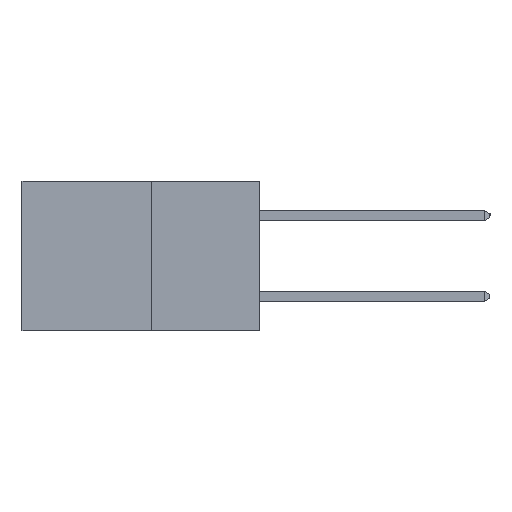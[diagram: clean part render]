
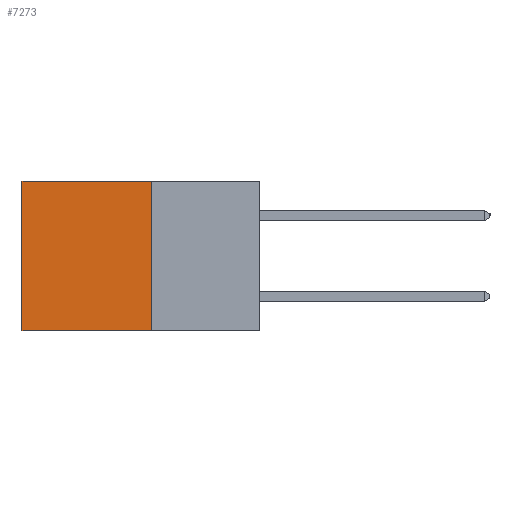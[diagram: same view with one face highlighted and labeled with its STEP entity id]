
A CAD part, left-side view. The second image highlights one B-rep face of the part: STEP entity #7273.
In plain terms, the highlighted planar face has unit normal (-1, 0, 0).
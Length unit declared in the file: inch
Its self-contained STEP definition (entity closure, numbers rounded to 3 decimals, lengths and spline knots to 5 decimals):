
#501 = LINE ( 'NONE', #6495, #8125 ) ;
#577 = VERTEX_POINT ( 'NONE', #7725 ) ;
#674 = ORIENTED_EDGE ( 'NONE', *, *, #4969, .F. ) ;
#1508 = LINE ( 'NONE', #6036, #3295 ) ;
#1708 = FACE_OUTER_BOUND ( 'NONE', #6124, .T. ) ;
#1887 = CARTESIAN_POINT ( 'NONE',  ( 0.277, 0.27, -0.37 ) ) ;
#2261 = CARTESIAN_POINT ( 'NONE',  ( 0.277, 0.27, 0. ) ) ;
#2389 = ORIENTED_EDGE ( 'NONE', *, *, #8912, .T. ) ;
#2545 = VERTEX_POINT ( 'NONE', #6766 ) ;
#2598 = DIRECTION ( 'NONE',  ( 1., 0., 0. ) ) ;
#2886 = PLANE ( 'NONE',  #6921 ) ;
#3295 = VECTOR ( 'NONE', #4613, 39.37008 ) ;
#3576 = CARTESIAN_POINT ( 'NONE',  ( 0.277, 0.59, 0. ) ) ;
#3911 = ORIENTED_EDGE ( 'NONE', *, *, #4428, .T. ) ;
#3954 = ORIENTED_EDGE ( 'NONE', *, *, #8108, .F. ) ;
#4246 = DIRECTION ( 'NONE',  ( 0., 1., 0. ) ) ;
#4428 = EDGE_CURVE ( 'NONE', #7630, #2545, #1508, .T. ) ;
#4613 = DIRECTION ( 'NONE',  ( 0., 0., -1. ) ) ;
#4969 = EDGE_CURVE ( 'NONE', #6392, #577, #8289, .T. ) ;
#5275 = CARTESIAN_POINT ( 'NONE',  ( 0.277, 0.27, 0. ) ) ;
#5838 = DIRECTION ( 'NONE',  ( 0., 0., -1. ) ) ;
#6036 = CARTESIAN_POINT ( 'NONE',  ( 0.277, 0.59, -0.37 ) ) ;
#6109 = CARTESIAN_POINT ( 'NONE',  ( 0.277, 0.27, -0.37 ) ) ;
#6124 = EDGE_LOOP ( 'NONE', ( #3911, #3954, #674, #2389 ) ) ;
#6392 = VERTEX_POINT ( 'NONE', #5275 ) ;
#6495 = CARTESIAN_POINT ( 'NONE',  ( 0.277, 0.27, -0.37 ) ) ;
#6766 = CARTESIAN_POINT ( 'NONE',  ( 0.277, 0.59, -0.37 ) ) ;
#6921 = AXIS2_PLACEMENT_3D ( 'NONE', #1887, #2598, #6967 ) ;
#6967 = DIRECTION ( 'NONE',  ( 0., 0., -1. ) ) ;
#7273 = ADVANCED_FACE ( 'NONE', ( #1708 ), #2886, .F. ) ;
#7487 = VECTOR ( 'NONE', #7615, 39.37008 ) ;
#7615 = DIRECTION ( 'NONE',  ( 0., 1., 0. ) ) ;
#7630 = VERTEX_POINT ( 'NONE', #3576 ) ;
#7725 = CARTESIAN_POINT ( 'NONE',  ( 0.277, 0.27, -0.37 ) ) ;
#8079 = VECTOR ( 'NONE', #5838, 39.37008 ) ;
#8108 = EDGE_CURVE ( 'NONE', #577, #2545, #501, .T. ) ;
#8125 = VECTOR ( 'NONE', #4246, 39.37008 ) ;
#8289 = LINE ( 'NONE', #6109, #8079 ) ;
#8912 = EDGE_CURVE ( 'NONE', #6392, #7630, #9264, .T. ) ;
#9264 = LINE ( 'NONE', #2261, #7487 ) ;
